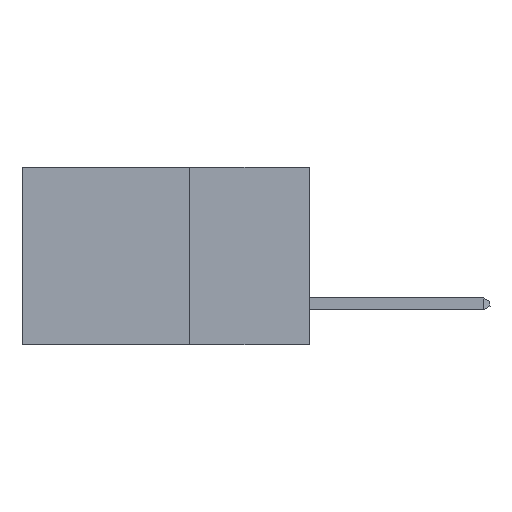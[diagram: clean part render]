
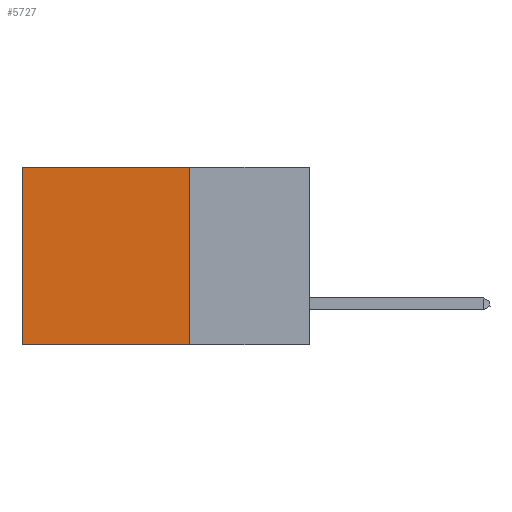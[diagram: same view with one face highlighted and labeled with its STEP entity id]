
A CAD part, left-side view. The second image highlights one B-rep face of the part: STEP entity #5727.
In plain terms, the highlighted planar face has unit normal (-1, 0, 0).
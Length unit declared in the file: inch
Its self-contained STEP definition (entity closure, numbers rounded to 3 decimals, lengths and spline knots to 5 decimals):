
#69 = VECTOR ( 'NONE', #13124, 39.37008 ) ;
#445 = LINE ( 'NONE', #6847, #69 ) ;
#710 = CARTESIAN_POINT ( 'NONE',  ( 0.2875, 0.25, -0.37 ) ) ;
#935 = CARTESIAN_POINT ( 'NONE',  ( 0.2875, 0.25, -0.37 ) ) ;
#1014 = CARTESIAN_POINT ( 'NONE',  ( 0.2875, 0.6, -0.37 ) ) ;
#1396 = DIRECTION ( 'NONE',  ( 0., 0., -1. ) ) ;
#1965 = VERTEX_POINT ( 'NONE', #1014 ) ;
#2346 = FACE_OUTER_BOUND ( 'NONE', #7158, .T. ) ;
#3313 = VERTEX_POINT ( 'NONE', #4592 ) ;
#4227 = ORIENTED_EDGE ( 'NONE', *, *, #10121, .F. ) ;
#4389 = VECTOR ( 'NONE', #1396, 39.37008 ) ;
#4467 = PLANE ( 'NONE',  #5362 ) ;
#4511 = CARTESIAN_POINT ( 'NONE',  ( 0.2875, 0.6, 0. ) ) ;
#4592 = CARTESIAN_POINT ( 'NONE',  ( 0.2875, 0.25, 0. ) ) ;
#5362 = AXIS2_PLACEMENT_3D ( 'NONE', #11975, #5576, #12978 ) ;
#5404 = VECTOR ( 'NONE', #9865, 39.37008 ) ;
#5576 = DIRECTION ( 'NONE',  ( 1., 0., 0. ) ) ;
#5699 = EDGE_CURVE ( 'NONE', #3313, #10910, #11128, .T. ) ;
#5727 = ADVANCED_FACE ( 'NONE', ( #2346 ), #4467, .F. ) ;
#6847 = CARTESIAN_POINT ( 'NONE',  ( 0.2875, 0.25, 0. ) ) ;
#7158 = EDGE_LOOP ( 'NONE', ( #14193, #4227, #8687, #8727 ) ) ;
#7676 = DIRECTION ( 'NONE',  ( 0., 1., 0. ) ) ;
#8687 = ORIENTED_EDGE ( 'NONE', *, *, #5699, .F. ) ;
#8727 = ORIENTED_EDGE ( 'NONE', *, *, #9667, .T. ) ;
#9337 = CARTESIAN_POINT ( 'NONE',  ( 0.2875, 0.6, 0. ) ) ;
#9573 = VECTOR ( 'NONE', #7676, 39.37008 ) ;
#9667 = EDGE_CURVE ( 'NONE', #3313, #12594, #445, .T. ) ;
#9817 = CARTESIAN_POINT ( 'NONE',  ( 0.2875, 0.25, 0. ) ) ;
#9865 = DIRECTION ( 'NONE',  ( 0., 0., -1. ) ) ;
#10121 = EDGE_CURVE ( 'NONE', #10910, #1965, #12614, .T. ) ;
#10910 = VERTEX_POINT ( 'NONE', #935 ) ;
#11128 = LINE ( 'NONE', #9817, #5404 ) ;
#11716 = EDGE_CURVE ( 'NONE', #12594, #1965, #12884, .T. ) ;
#11975 = CARTESIAN_POINT ( 'NONE',  ( 0.2875, 0.25, 0. ) ) ;
#12594 = VERTEX_POINT ( 'NONE', #4511 ) ;
#12614 = LINE ( 'NONE', #710, #9573 ) ;
#12884 = LINE ( 'NONE', #9337, #4389 ) ;
#12978 = DIRECTION ( 'NONE',  ( 0., 0., -1. ) ) ;
#13124 = DIRECTION ( 'NONE',  ( 0., 1., 0. ) ) ;
#14193 = ORIENTED_EDGE ( 'NONE', *, *, #11716, .T. ) ;
